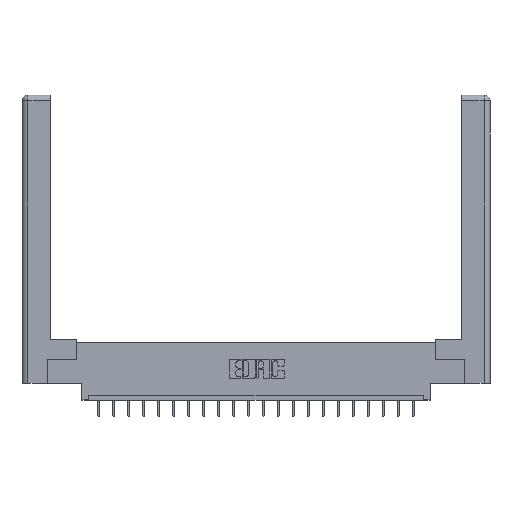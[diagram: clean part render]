
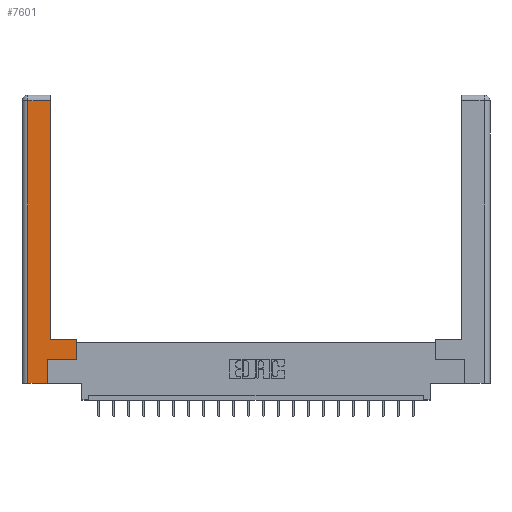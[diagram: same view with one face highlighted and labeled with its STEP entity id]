
A CAD part, top view. The second image highlights one B-rep face of the part: STEP entity #7601.
In plain terms, the highlighted planar face has unit normal (0, 0, 1).
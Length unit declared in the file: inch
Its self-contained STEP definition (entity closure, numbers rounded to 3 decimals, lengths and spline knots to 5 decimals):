
#91 = ORIENTED_EDGE ( 'NONE', *, *, #1432, .T. ) ;
#110 = EDGE_CURVE ( 'NONE', #16045, #6596, #15774, .T. ) ;
#982 = DIRECTION ( 'NONE',  ( 0., 0., -1. ) ) ;
#1144 = EDGE_CURVE ( 'NONE', #9055, #2278, #5407, .T. ) ;
#1183 = DIRECTION ( 'NONE',  ( -1., 0., 0. ) ) ;
#1390 = VECTOR ( 'NONE', #20736, 39.37008 ) ;
#1432 = EDGE_CURVE ( 'NONE', #6596, #2269, #18072, .T. ) ;
#1443 = CARTESIAN_POINT ( 'NONE',  ( 0.295, 0.45, 0. ) ) ;
#1503 = VERTEX_POINT ( 'NONE', #21400 ) ;
#2118 = CARTESIAN_POINT ( 'NONE',  ( 0.565, 0.45, 0. ) ) ;
#2269 = VERTEX_POINT ( 'NONE', #20457 ) ;
#2278 = VERTEX_POINT ( 'NONE', #2118 ) ;
#2805 = CARTESIAN_POINT ( 'NONE',  ( 0., 0., 0. ) ) ;
#3353 = DIRECTION ( 'NONE',  ( 0., 1., 0. ) ) ;
#3500 = EDGE_CURVE ( 'NONE', #2269, #9055, #5834, .T. ) ;
#3619 = EDGE_CURVE ( 'NONE', #15141, #1503, #20095, .T. ) ;
#4139 = VECTOR ( 'NONE', #19993, 39.37008 ) ;
#4303 = EDGE_CURVE ( 'NONE', #2278, #13351, #18760, .T. ) ;
#4667 = CARTESIAN_POINT ( 'NONE',  ( 0.265, 0.245, 0. ) ) ;
#5135 = LINE ( 'NONE', #11337, #10185 ) ;
#5407 = LINE ( 'NONE', #6496, #20194 ) ;
#5834 = LINE ( 'NONE', #12507, #1390 ) ;
#6075 = EDGE_LOOP ( 'NONE', ( #18025, #7038, #7544, #15089, #91, #19155, #11670, #21556 ) ) ;
#6282 = DIRECTION ( 'NONE',  ( 0., 1., 0. ) ) ;
#6496 = CARTESIAN_POINT ( 'NONE',  ( 0.565, 0.45, 0. ) ) ;
#6596 = VERTEX_POINT ( 'NONE', #16629 ) ;
#7007 = EDGE_CURVE ( 'NONE', #1503, #16045, #16023, .T. ) ;
#7018 = FACE_OUTER_BOUND ( 'NONE', #6075, .T. ) ;
#7038 = ORIENTED_EDGE ( 'NONE', *, *, #3619, .T. ) ;
#7523 = EDGE_CURVE ( 'NONE', #13351, #15141, #5135, .T. ) ;
#7544 = ORIENTED_EDGE ( 'NONE', *, *, #7007, .T. ) ;
#7601 = ADVANCED_FACE ( 'NONE', ( #7018 ), #21419, .F. ) ;
#8204 = CARTESIAN_POINT ( 'NONE',  ( 0.0615, 0., 0. ) ) ;
#9055 = VERTEX_POINT ( 'NONE', #13787 ) ;
#9081 = VECTOR ( 'NONE', #16498, 39.37008 ) ;
#10185 = VECTOR ( 'NONE', #6282, 39.37008 ) ;
#10657 = CARTESIAN_POINT ( 'NONE',  ( 0.0615, 0., 0. ) ) ;
#11337 = CARTESIAN_POINT ( 'NONE',  ( 0.295, 3., 0. ) ) ;
#11670 = ORIENTED_EDGE ( 'NONE', *, *, #1144, .T. ) ;
#12507 = CARTESIAN_POINT ( 'NONE',  ( 0.565, 0.245, 0. ) ) ;
#13351 = VERTEX_POINT ( 'NONE', #1443 ) ;
#13782 = DIRECTION ( 'NONE',  ( 1., 0., 0. ) ) ;
#13787 = CARTESIAN_POINT ( 'NONE',  ( 0.565, 0.245, 0. ) ) ;
#14765 = CARTESIAN_POINT ( 'NONE',  ( 0.0615, 2.94, 0. ) ) ;
#15089 = ORIENTED_EDGE ( 'NONE', *, *, #110, .T. ) ;
#15141 = VERTEX_POINT ( 'NONE', #21181 ) ;
#15631 = VECTOR ( 'NONE', #1183, 39.37008 ) ;
#15774 = LINE ( 'NONE', #17105, #17881 ) ;
#16023 = LINE ( 'NONE', #8204, #4139 ) ;
#16045 = VERTEX_POINT ( 'NONE', #10657 ) ;
#16498 = DIRECTION ( 'NONE',  ( 0., 1., 0. ) ) ;
#16629 = CARTESIAN_POINT ( 'NONE',  ( 0.265, 0., 0. ) ) ;
#17105 = CARTESIAN_POINT ( 'NONE',  ( 0.265, 0., 0. ) ) ;
#17170 = CARTESIAN_POINT ( 'NONE',  ( 0.295, 0.45, 0. ) ) ;
#17451 = VECTOR ( 'NONE', #20746, 39.37008 ) ;
#17881 = VECTOR ( 'NONE', #13782, 39.37008 ) ;
#18025 = ORIENTED_EDGE ( 'NONE', *, *, #7523, .T. ) ;
#18072 = LINE ( 'NONE', #4667, #9081 ) ;
#18760 = LINE ( 'NONE', #17170, #17451 ) ;
#19155 = ORIENTED_EDGE ( 'NONE', *, *, #3500, .T. ) ;
#19993 = DIRECTION ( 'NONE',  ( 0., -1., 0. ) ) ;
#20095 = LINE ( 'NONE', #14765, #15631 ) ;
#20194 = VECTOR ( 'NONE', #3353, 39.37008 ) ;
#20457 = CARTESIAN_POINT ( 'NONE',  ( 0.265, 0.245, 0. ) ) ;
#20736 = DIRECTION ( 'NONE',  ( 1., 0., 0. ) ) ;
#20746 = DIRECTION ( 'NONE',  ( -1., 0., 0. ) ) ;
#21043 = AXIS2_PLACEMENT_3D ( 'NONE', #2805, #982, #21345 ) ;
#21181 = CARTESIAN_POINT ( 'NONE',  ( 0.295, 2.94, 0. ) ) ;
#21345 = DIRECTION ( 'NONE',  ( -1., 0., 0. ) ) ;
#21400 = CARTESIAN_POINT ( 'NONE',  ( 0.0615, 2.94, 0. ) ) ;
#21419 = PLANE ( 'NONE',  #21043 ) ;
#21556 = ORIENTED_EDGE ( 'NONE', *, *, #4303, .T. ) ;
